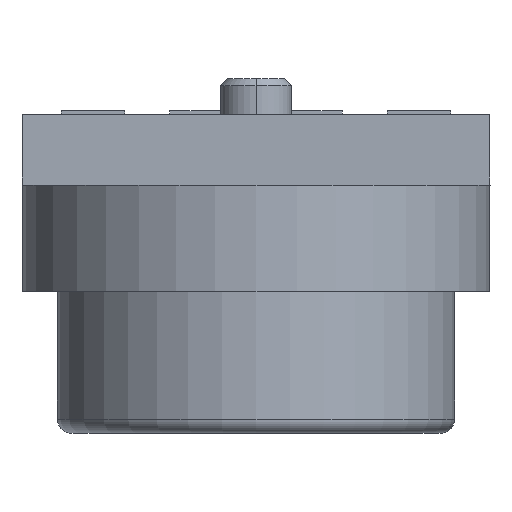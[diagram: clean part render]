
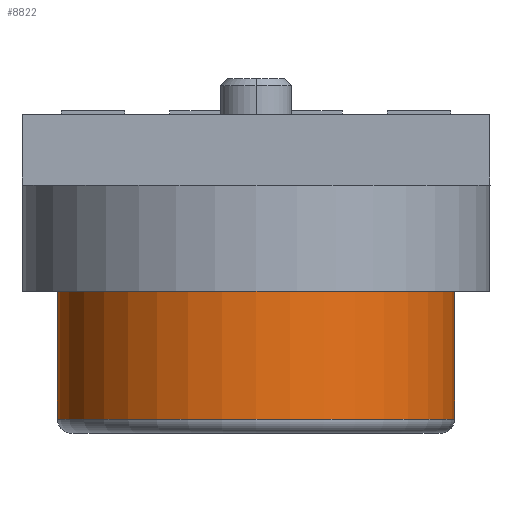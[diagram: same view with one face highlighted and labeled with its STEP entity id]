
A CAD part, left-side view. The second image highlights one B-rep face of the part: STEP entity #8822.
In plain terms, the highlighted cylindrical face has radius 2.8 mm (diameter 5.6 mm), a partial arc.
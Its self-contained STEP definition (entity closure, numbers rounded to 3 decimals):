
#307 = CIRCLE ( 'NONE', #9563, 2.8 ) ;
#423 = DIRECTION ( 'NONE',  ( 0., 0., -1. ) ) ;
#1029 = CYLINDRICAL_SURFACE ( 'NONE', #9005, 2.8 ) ;
#1384 = CARTESIAN_POINT ( 'NONE',  ( -8.63, -2.8, 7.2 ) ) ;
#1597 = LINE ( 'NONE', #4920, #3253 ) ;
#1703 = DIRECTION ( 'NONE',  ( 0., 0., -1. ) ) ;
#2102 = CARTESIAN_POINT ( 'NONE',  ( -8.63, 2.8, 9. ) ) ;
#2220 = ORIENTED_EDGE ( 'NONE', *, *, #10371, .F. ) ;
#2524 = VERTEX_POINT ( 'NONE', #1384 ) ;
#2597 = EDGE_CURVE ( 'NONE', #4590, #2524, #1597, .T. ) ;
#2752 = DIRECTION ( 'NONE',  ( 1., 0., 0. ) ) ;
#2882 = CARTESIAN_POINT ( 'NONE',  ( -8.63, 0., 7.2 ) ) ;
#3253 = VECTOR ( 'NONE', #1703, 1000. ) ;
#3900 = EDGE_CURVE ( 'NONE', #4590, #10736, #8172, .T. ) ;
#3960 = EDGE_CURVE ( 'NONE', #9489, #2524, #307, .T. ) ;
#3983 = AXIS2_PLACEMENT_3D ( 'NONE', #4476, #9671, #6245 ) ;
#4476 = CARTESIAN_POINT ( 'NONE',  ( -8.63, 0., 9. ) ) ;
#4580 = DIRECTION ( 'NONE',  ( 0., 0., 1. ) ) ;
#4590 = VERTEX_POINT ( 'NONE', #9737 ) ;
#4920 = CARTESIAN_POINT ( 'NONE',  ( -8.63, -2.8, 9. ) ) ;
#5859 = CARTESIAN_POINT ( 'NONE',  ( -8.63, 2.8, 7.2 ) ) ;
#6097 = LINE ( 'NONE', #9420, #8736 ) ;
#6150 = ORIENTED_EDGE ( 'NONE', *, *, #2597, .F. ) ;
#6245 = DIRECTION ( 'NONE',  ( 0., -1., 0. ) ) ;
#6605 = ORIENTED_EDGE ( 'NONE', *, *, #3960, .T. ) ;
#8172 = CIRCLE ( 'NONE', #3983, 2.8 ) ;
#8686 = DIRECTION ( 'NONE',  ( -0.013, -1., 0. ) ) ;
#8736 = VECTOR ( 'NONE', #10334, 1000. ) ;
#8822 = ADVANCED_FACE ( 'NONE', ( #9343 ), #1029, .T. ) ;
#9005 = AXIS2_PLACEMENT_3D ( 'NONE', #10423, #423, #2752 ) ;
#9343 = FACE_OUTER_BOUND ( 'NONE', #9434, .T. ) ;
#9420 = CARTESIAN_POINT ( 'NONE',  ( -8.63, 2.8, 7.2 ) ) ;
#9434 = EDGE_LOOP ( 'NONE', ( #6150, #10170, #2220, #6605 ) ) ;
#9489 = VERTEX_POINT ( 'NONE', #5859 ) ;
#9563 = AXIS2_PLACEMENT_3D ( 'NONE', #2882, #4580, #8686 ) ;
#9671 = DIRECTION ( 'NONE',  ( 0., 0., -1. ) ) ;
#9737 = CARTESIAN_POINT ( 'NONE',  ( -8.63, -2.8, 9. ) ) ;
#10170 = ORIENTED_EDGE ( 'NONE', *, *, #3900, .T. ) ;
#10334 = DIRECTION ( 'NONE',  ( 0., 0., 1. ) ) ;
#10371 = EDGE_CURVE ( 'NONE', #9489, #10736, #6097, .T. ) ;
#10423 = CARTESIAN_POINT ( 'NONE',  ( -8.63, 0., 9.036 ) ) ;
#10736 = VERTEX_POINT ( 'NONE', #2102 ) ;
